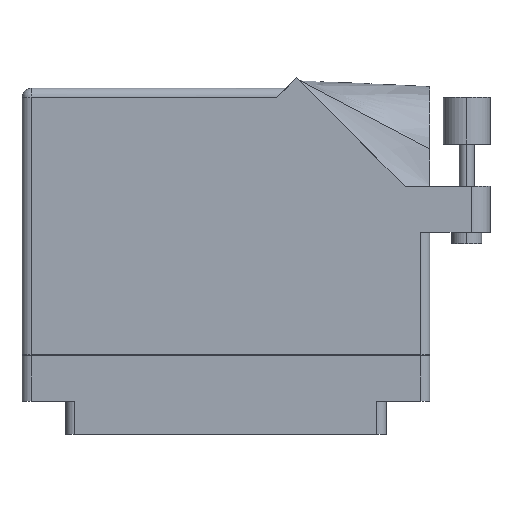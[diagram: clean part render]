
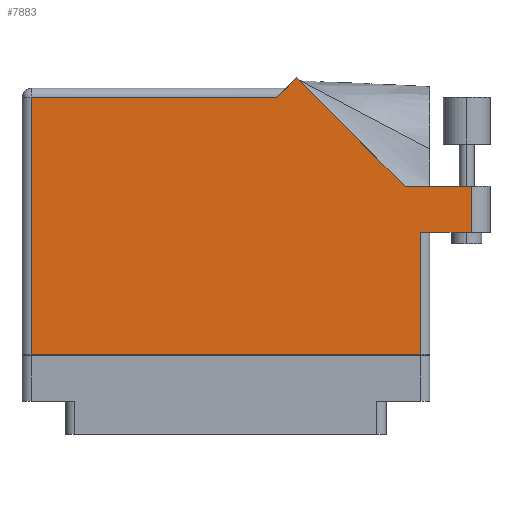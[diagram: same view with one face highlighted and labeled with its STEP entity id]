
A CAD part, front view. The second image highlights one B-rep face of the part: STEP entity #7883.
In plain terms, the highlighted face is planar.
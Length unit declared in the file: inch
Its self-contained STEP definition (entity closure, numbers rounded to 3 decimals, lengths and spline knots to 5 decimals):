
#156 = CARTESIAN_POINT ( 'NONE',  ( 1.19342, 1.022, 0.617 ) ) ;
#332 = LINE ( 'NONE', #56690, #9761 ) ;
#3127 = DIRECTION ( 'NONE',  ( 0., -1., 0. ) ) ;
#3431 = ORIENTED_EDGE ( 'NONE', *, *, #29401, .T. ) ;
#5074 = VECTOR ( 'NONE', #15880, 39.37008 ) ;
#6788 = EDGE_CURVE ( 'NONE', #42067, #37917, #59721, .T. ) ;
#7299 = EDGE_CURVE ( 'NONE', #35993, #60870, #63582, .T. ) ;
#7883 = ADVANCED_FACE ( 'NONE', ( #29783 ), #38930, .F. ) ;
#8199 = VECTOR ( 'NONE', #15522, 39.37008 ) ;
#8201 = EDGE_LOOP ( 'NONE', ( #44620, #40121, #60347, #16569, #3431, #61787, #39933, #63748, #49284 ) ) ;
#8231 = CARTESIAN_POINT ( 'NONE',  ( -1.297, -0.1, 0.617 ) ) ;
#9215 = CARTESIAN_POINT ( 'NONE',  ( 1.19342, 1.022, 0.617 ) ) ;
#9761 = VECTOR ( 'NONE', #62350, 39.37008 ) ;
#9826 = LINE ( 'NONE', #10027, #5074 ) ;
#10027 = CARTESIAN_POINT ( 'NONE',  ( 1.634, 1.022, 0.617 ) ) ;
#10595 = CARTESIAN_POINT ( 'NONE',  ( -1.359, 1.675, 0.617 ) ) ;
#12335 = CARTESIAN_POINT ( 'NONE',  ( -1.297, -0.1, 0.617 ) ) ;
#12879 = EDGE_CURVE ( 'NONE', #51968, #42067, #9826, .T. ) ;
#14133 = AXIS2_PLACEMENT_3D ( 'NONE', #10595, #50477, #60479 ) ;
#15522 = DIRECTION ( 'NONE',  ( 1., 0., 0. ) ) ;
#15880 = DIRECTION ( 'NONE',  ( 0., 1., 0. ) ) ;
#16189 = VERTEX_POINT ( 'NONE', #47916 ) ;
#16569 = ORIENTED_EDGE ( 'NONE', *, *, #31513, .T. ) ;
#17735 = CARTESIAN_POINT ( 'NONE',  ( -1.359, 1.613, 0.617 ) ) ;
#19961 = CARTESIAN_POINT ( 'NONE',  ( -1.359, -0.1, 0.617 ) ) ;
#20653 = DIRECTION ( 'NONE',  ( -1., 0., 0. ) ) ;
#21630 = EDGE_CURVE ( 'NONE', #60870, #46176, #332, .T. ) ;
#23929 = CARTESIAN_POINT ( 'NONE',  ( 0.46971, 1.74571, 0.617 ) ) ;
#25016 = LINE ( 'NONE', #17735, #64762 ) ;
#26263 = LINE ( 'NONE', #53825, #60505 ) ;
#29401 = EDGE_CURVE ( 'NONE', #31040, #16189, #42529, .T. ) ;
#29783 = FACE_OUTER_BOUND ( 'NONE', #8201, .T. ) ;
#31040 = VERTEX_POINT ( 'NONE', #23929 ) ;
#31513 = EDGE_CURVE ( 'NONE', #37917, #31040, #42969, .T. ) ;
#32053 = CARTESIAN_POINT ( 'NONE',  ( 1.297, 0.715, 0.617 ) ) ;
#33845 = CARTESIAN_POINT ( 'NONE',  ( 1.634, 0.715, 0.617 ) ) ;
#33955 = LINE ( 'NONE', #12335, #59693 ) ;
#35198 = VECTOR ( 'NONE', #63696, 39.37008 ) ;
#35993 = VERTEX_POINT ( 'NONE', #8231 ) ;
#36191 = CARTESIAN_POINT ( 'NONE',  ( 1.634, 1.022, 0.617 ) ) ;
#37169 = CARTESIAN_POINT ( 'NONE',  ( 0.399, 1.675, 0.617 ) ) ;
#37917 = VERTEX_POINT ( 'NONE', #9215 ) ;
#38930 = PLANE ( 'NONE',  #14133 ) ;
#39933 = ORIENTED_EDGE ( 'NONE', *, *, #56717, .T. ) ;
#40121 = ORIENTED_EDGE ( 'NONE', *, *, #12879, .T. ) ;
#40437 = CARTESIAN_POINT ( 'NONE',  ( 1.759, 1.022, 0.617 ) ) ;
#41973 = DIRECTION ( 'NONE',  ( -0.707, -0.707, 0. ) ) ;
#42067 = VERTEX_POINT ( 'NONE', #36191 ) ;
#42529 = LINE ( 'NONE', #37169, #56563 ) ;
#42969 = LINE ( 'NONE', #156, #35198 ) ;
#44620 = ORIENTED_EDGE ( 'NONE', *, *, #56328, .T. ) ;
#46176 = VERTEX_POINT ( 'NONE', #32053 ) ;
#46470 = VECTOR ( 'NONE', #20653, 39.37008 ) ;
#47393 = DIRECTION ( 'NONE',  ( -1., 0., 0. ) ) ;
#47889 = CARTESIAN_POINT ( 'NONE',  ( 1.297, -0.1, 0.617 ) ) ;
#47916 = CARTESIAN_POINT ( 'NONE',  ( 0.337, 1.613, 0.617 ) ) ;
#49284 = ORIENTED_EDGE ( 'NONE', *, *, #21630, .T. ) ;
#50337 = EDGE_CURVE ( 'NONE', #16189, #60596, #25016, .T. ) ;
#50477 = DIRECTION ( 'NONE',  ( 0., 0., -1. ) ) ;
#51968 = VERTEX_POINT ( 'NONE', #33845 ) ;
#53825 = CARTESIAN_POINT ( 'NONE',  ( 1.359, 0.715, 0.617 ) ) ;
#56133 = CARTESIAN_POINT ( 'NONE',  ( -1.297, 1.613, 0.617 ) ) ;
#56328 = EDGE_CURVE ( 'NONE', #46176, #51968, #26263, .T. ) ;
#56563 = VECTOR ( 'NONE', #41973, 39.37008 ) ;
#56690 = CARTESIAN_POINT ( 'NONE',  ( 1.297, 0.715, 0.617 ) ) ;
#56717 = EDGE_CURVE ( 'NONE', #60596, #35993, #33955, .T. ) ;
#59693 = VECTOR ( 'NONE', #3127, 39.37008 ) ;
#59721 = LINE ( 'NONE', #40437, #46470 ) ;
#60347 = ORIENTED_EDGE ( 'NONE', *, *, #6788, .T. ) ;
#60479 = DIRECTION ( 'NONE',  ( -1., 0., 0. ) ) ;
#60505 = VECTOR ( 'NONE', #63438, 39.37008 ) ;
#60596 = VERTEX_POINT ( 'NONE', #56133 ) ;
#60870 = VERTEX_POINT ( 'NONE', #47889 ) ;
#61787 = ORIENTED_EDGE ( 'NONE', *, *, #50337, .T. ) ;
#62350 = DIRECTION ( 'NONE',  ( 0., 1., 0. ) ) ;
#63438 = DIRECTION ( 'NONE',  ( 1., 0., 0. ) ) ;
#63582 = LINE ( 'NONE', #19961, #8199 ) ;
#63696 = DIRECTION ( 'NONE',  ( -0.707, 0.707, 0. ) ) ;
#63748 = ORIENTED_EDGE ( 'NONE', *, *, #7299, .T. ) ;
#64762 = VECTOR ( 'NONE', #47393, 39.37008 ) ;
